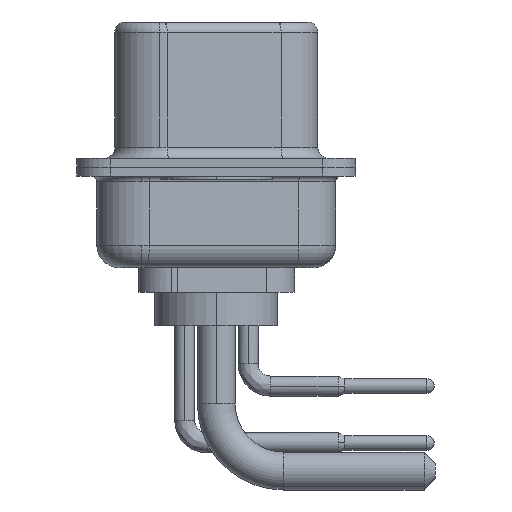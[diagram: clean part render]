
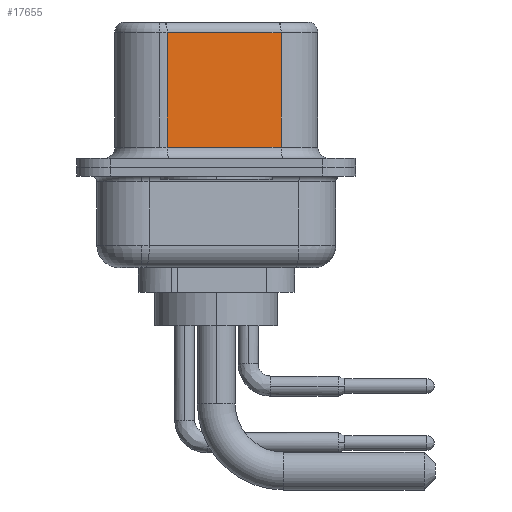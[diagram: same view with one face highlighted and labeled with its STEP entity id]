
A CAD part, left-side view. The second image highlights one B-rep face of the part: STEP entity #17655.
In plain terms, the highlighted planar face has unit normal (-0.985, -0.174, 0).
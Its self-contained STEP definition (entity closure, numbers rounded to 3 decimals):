
#71 = VECTOR ( 'NONE', #13229, 1000. ) ;
#2430 = LINE ( 'NONE', #7943, #23934 ) ;
#2693 = EDGE_CURVE ( 'NONE', #20303, #18757, #22822, .T. ) ;
#3687 = DIRECTION ( 'NONE',  ( -0.174, 0.985, 0. ) ) ;
#4167 = FACE_OUTER_BOUND ( 'NONE', #10581, .T. ) ;
#4670 = CARTESIAN_POINT ( 'NONE',  ( 4.58, -2.897, 6.02 ) ) ;
#5487 = EDGE_CURVE ( 'NONE', #20800, #6615, #6216, .T. ) ;
#5913 = PLANE ( 'NONE',  #12402 ) ;
#6216 = LINE ( 'NONE', #16362, #9410 ) ;
#6615 = VERTEX_POINT ( 'NONE', #8329 ) ;
#6712 = DIRECTION ( 'NONE',  ( 0., 0., -1. ) ) ;
#7421 = CARTESIAN_POINT ( 'NONE',  ( 4.58, -2.897, 6.02 ) ) ;
#7608 = ORIENTED_EDGE ( 'NONE', *, *, #13348, .T. ) ;
#7676 = CARTESIAN_POINT ( 'NONE',  ( 4.58, -2.897, 0.9 ) ) ;
#7943 = CARTESIAN_POINT ( 'NONE',  ( 4.58, -2.897, 0.9 ) ) ;
#8329 = CARTESIAN_POINT ( 'NONE',  ( 3.68, 2.203, 0.9 ) ) ;
#9407 = ORIENTED_EDGE ( 'NONE', *, *, #5487, .T. ) ;
#9410 = VECTOR ( 'NONE', #6712, 1000. ) ;
#10581 = EDGE_LOOP ( 'NONE', ( #16989, #14308, #9407, #7608 ) ) ;
#11207 = DIRECTION ( 'NONE',  ( -0.174, 0.985, 0. ) ) ;
#12402 = AXIS2_PLACEMENT_3D ( 'NONE', #20980, #15430, #3687 ) ;
#13063 = CARTESIAN_POINT ( 'NONE',  ( 3.68, 2.203, 6.02 ) ) ;
#13229 = DIRECTION ( 'NONE',  ( 0., 0., -1. ) ) ;
#13348 = EDGE_CURVE ( 'NONE', #6615, #18757, #2430, .T. ) ;
#14308 = ORIENTED_EDGE ( 'NONE', *, *, #24665, .T. ) ;
#15430 = DIRECTION ( 'NONE',  ( 0.985, 0.174, 0. ) ) ;
#16362 = CARTESIAN_POINT ( 'NONE',  ( 3.68, 2.203, 6.52 ) ) ;
#16989 = ORIENTED_EDGE ( 'NONE', *, *, #2693, .F. ) ;
#17655 = ADVANCED_FACE ( 'NONE', ( #4167 ), #5913, .F. ) ;
#18757 = VERTEX_POINT ( 'NONE', #7676 ) ;
#18815 = VECTOR ( 'NONE', #11207, 1000. ) ;
#18842 = LINE ( 'NONE', #7421, #18815 ) ;
#20303 = VERTEX_POINT ( 'NONE', #4670 ) ;
#20800 = VERTEX_POINT ( 'NONE', #13063 ) ;
#20980 = CARTESIAN_POINT ( 'NONE',  ( 4.58, -2.897, 6.52 ) ) ;
#22822 = LINE ( 'NONE', #22949, #71 ) ;
#22949 = CARTESIAN_POINT ( 'NONE',  ( 4.58, -2.897, 6.52 ) ) ;
#23134 = DIRECTION ( 'NONE',  ( 0.174, -0.985, 0. ) ) ;
#23934 = VECTOR ( 'NONE', #23134, 1000. ) ;
#24665 = EDGE_CURVE ( 'NONE', #20303, #20800, #18842, .T. ) ;
